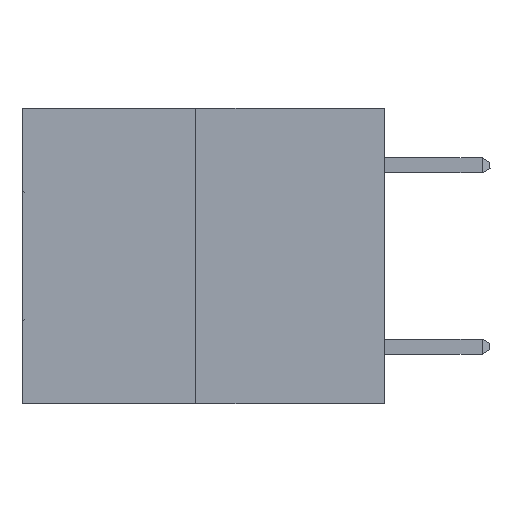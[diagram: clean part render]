
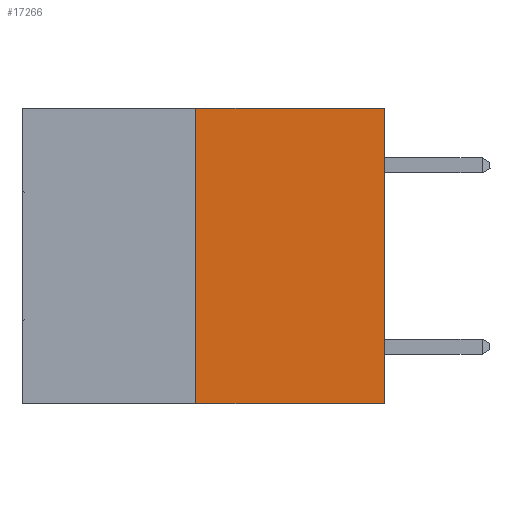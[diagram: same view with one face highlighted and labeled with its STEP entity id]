
A CAD part, left-side view. The second image highlights one B-rep face of the part: STEP entity #17266.
In plain terms, the highlighted planar face has unit normal (-1, 0, 0).
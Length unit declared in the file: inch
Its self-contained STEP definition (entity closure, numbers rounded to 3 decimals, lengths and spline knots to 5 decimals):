
#1198 = CARTESIAN_POINT ( 'NONE',  ( 0., 0., 0. ) ) ;
#1315 = CARTESIAN_POINT ( 'NONE',  ( 0., 0., -0.49 ) ) ;
#3346 = CARTESIAN_POINT ( 'NONE',  ( 0., 0.6, -0.49 ) ) ;
#4815 = CARTESIAN_POINT ( 'NONE',  ( 0., 0.6, 0. ) ) ;
#4997 = EDGE_CURVE ( 'NONE', #21611, #29761, #35394, .T. ) ;
#5096 = ORIENTED_EDGE ( 'NONE', *, *, #4997, .T. ) ;
#5632 = EDGE_CURVE ( 'NONE', #21611, #12615, #22982, .T. ) ;
#6695 = VECTOR ( 'NONE', #23328, 39.37008 ) ;
#9461 = CARTESIAN_POINT ( 'NONE',  ( 0., 0.312, 0. ) ) ;
#9568 = CARTESIAN_POINT ( 'NONE',  ( 0., 0.312, -0.49 ) ) ;
#10161 = VECTOR ( 'NONE', #20371, 39.37008 ) ;
#11425 = ORIENTED_EDGE ( 'NONE', *, *, #5632, .F. ) ;
#11630 = VERTEX_POINT ( 'NONE', #27613 ) ;
#11787 = DIRECTION ( 'NONE',  ( 0., -1., 0. ) ) ;
#12615 = VERTEX_POINT ( 'NONE', #9461 ) ;
#13533 = FACE_OUTER_BOUND ( 'NONE', #18950, .T. ) ;
#15629 = CARTESIAN_POINT ( 'NONE',  ( 0., 0.6, 0. ) ) ;
#16197 = VECTOR ( 'NONE', #18963, 39.37008 ) ;
#17266 = ADVANCED_FACE ( 'NONE', ( #13533 ), #34766, .F. ) ;
#17449 = LINE ( 'NONE', #1198, #10161 ) ;
#18378 = CARTESIAN_POINT ( 'NONE',  ( 0., 0.312, -0.49 ) ) ;
#18383 = DIRECTION ( 'NONE',  ( 0., 0., -1. ) ) ;
#18950 = EDGE_LOOP ( 'NONE', ( #11425, #5096, #27638, #19110 ) ) ;
#18963 = DIRECTION ( 'NONE',  ( 0., -1., 0. ) ) ;
#19110 = ORIENTED_EDGE ( 'NONE', *, *, #30293, .F. ) ;
#20371 = DIRECTION ( 'NONE',  ( 0., 0., 1. ) ) ;
#20869 = VECTOR ( 'NONE', #11787, 39.37008 ) ;
#21611 = VERTEX_POINT ( 'NONE', #18378 ) ;
#22982 = LINE ( 'NONE', #9568, #6695 ) ;
#23328 = DIRECTION ( 'NONE',  ( 0., 0., 1. ) ) ;
#25615 = EDGE_CURVE ( 'NONE', #29761, #11630, #17449, .T. ) ;
#27613 = CARTESIAN_POINT ( 'NONE',  ( 0., 0., 0. ) ) ;
#27638 = ORIENTED_EDGE ( 'NONE', *, *, #25615, .T. ) ;
#28502 = AXIS2_PLACEMENT_3D ( 'NONE', #15629, #34409, #18383 ) ;
#29761 = VERTEX_POINT ( 'NONE', #1315 ) ;
#29859 = LINE ( 'NONE', #4815, #16197 ) ;
#30293 = EDGE_CURVE ( 'NONE', #12615, #11630, #29859, .T. ) ;
#34409 = DIRECTION ( 'NONE',  ( 1., 0., 0. ) ) ;
#34766 = PLANE ( 'NONE',  #28502 ) ;
#35394 = LINE ( 'NONE', #3346, #20869 ) ;
